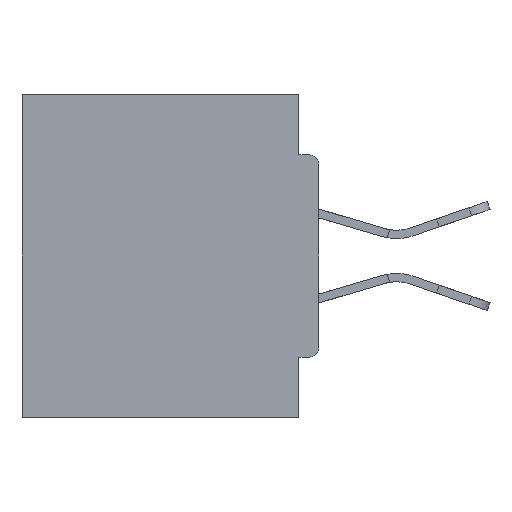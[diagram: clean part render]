
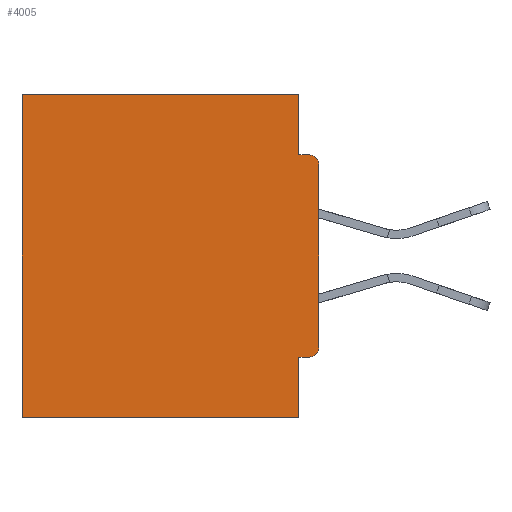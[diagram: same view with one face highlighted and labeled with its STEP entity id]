
A CAD part, left-side view. The second image highlights one B-rep face of the part: STEP entity #4005.
In plain terms, the highlighted planar face has unit normal (-1, 0, 0).
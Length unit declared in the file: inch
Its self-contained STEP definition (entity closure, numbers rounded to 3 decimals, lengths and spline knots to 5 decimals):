
#16 = DIRECTION ( 'NONE',  ( 1., 0., 0. ) ) ;
#240 = CIRCLE ( 'NONE', #25625, 0.015 ) ;
#1523 = LINE ( 'NONE', #36596, #21234 ) ;
#1583 = LINE ( 'NONE', #11855, #23850 ) ;
#2149 = LINE ( 'NONE', #12853, #18045 ) ;
#2560 = DIRECTION ( 'NONE',  ( -1., 0., 0. ) ) ;
#2942 = VERTEX_POINT ( 'NONE', #20227 ) ;
#3557 = CARTESIAN_POINT ( 'NONE',  ( 0.298, 0., 0. ) ) ;
#3755 = VERTEX_POINT ( 'NONE', #22875 ) ;
#3985 = CARTESIAN_POINT ( 'NONE',  ( 0.298, 0.031, -0.4065 ) ) ;
#4005 = ADVANCED_FACE ( 'NONE', ( #28245 ), #24340, .F. ) ;
#4211 = VECTOR ( 'NONE', #34764, 39.37008 ) ;
#5169 = VECTOR ( 'NONE', #29639, 39.37008 ) ;
#5307 = EDGE_CURVE ( 'NONE', #35157, #2942, #1583, .T. ) ;
#5792 = DIRECTION ( 'NONE',  ( 0., 0., -1. ) ) ;
#5953 = EDGE_CURVE ( 'NONE', #29725, #3755, #21306, .T. ) ;
#7488 = ORIENTED_EDGE ( 'NONE', *, *, #39979, .F. ) ;
#9000 = DIRECTION ( 'NONE',  ( 0., 1., 0. ) ) ;
#9446 = ORIENTED_EDGE ( 'NONE', *, *, #5953, .F. ) ;
#9539 = CARTESIAN_POINT ( 'NONE',  ( 0.298, 0.031, -0.5 ) ) ;
#11099 = CARTESIAN_POINT ( 'NONE',  ( 0.298, 0.031, -0.5 ) ) ;
#11128 = EDGE_CURVE ( 'NONE', #38319, #28306, #37104, .T. ) ;
#11855 = CARTESIAN_POINT ( 'NONE',  ( 0.298, 0., -0.5 ) ) ;
#12075 = DIRECTION ( 'NONE',  ( 0., 1., 0. ) ) ;
#12853 = CARTESIAN_POINT ( 'NONE',  ( 0.298, 0.46, 0. ) ) ;
#14094 = VECTOR ( 'NONE', #23771, 39.37008 ) ;
#14181 = VERTEX_POINT ( 'NONE', #31989 ) ;
#14245 = DIRECTION ( 'NONE',  ( -1., 0., 0. ) ) ;
#14380 = ORIENTED_EDGE ( 'NONE', *, *, #28101, .F. ) ;
#14704 = DIRECTION ( 'NONE',  ( 0., 0., -1. ) ) ;
#15812 = ORIENTED_EDGE ( 'NONE', *, *, #5307, .F. ) ;
#16065 = EDGE_CURVE ( 'NONE', #21220, #27363, #38179, .T. ) ;
#16906 = AXIS2_PLACEMENT_3D ( 'NONE', #31310, #2560, #34440 ) ;
#17268 = ORIENTED_EDGE ( 'NONE', *, *, #20866, .F. ) ;
#17435 = ORIENTED_EDGE ( 'NONE', *, *, #24050, .T. ) ;
#18045 = VECTOR ( 'NONE', #28828, 39.37008 ) ;
#18077 = LINE ( 'NONE', #20907, #26802 ) ;
#18659 = LINE ( 'NONE', #11099, #5169 ) ;
#19524 = DIRECTION ( 'NONE',  ( 0., 0., -1. ) ) ;
#19555 = CARTESIAN_POINT ( 'NONE',  ( 0.298, 0., -0.0935 ) ) ;
#20227 = CARTESIAN_POINT ( 'NONE',  ( 0.298, 0.46, -0.5 ) ) ;
#20441 = CARTESIAN_POINT ( 'NONE',  ( 0.298, 0.015, -0.1085 ) ) ;
#20866 = EDGE_CURVE ( 'NONE', #21220, #21267, #1523, .T. ) ;
#20907 = CARTESIAN_POINT ( 'NONE',  ( 0.298, 0.031, -0.5 ) ) ;
#21220 = VERTEX_POINT ( 'NONE', #22187 ) ;
#21234 = VECTOR ( 'NONE', #12075, 39.37008 ) ;
#21267 = VERTEX_POINT ( 'NONE', #3985 ) ;
#21306 = LINE ( 'NONE', #19555, #14094 ) ;
#22187 = CARTESIAN_POINT ( 'NONE',  ( 0.298, 0.015, -0.4065 ) ) ;
#22548 = CARTESIAN_POINT ( 'NONE',  ( 0.298, 0.46, 0. ) ) ;
#22875 = CARTESIAN_POINT ( 'NONE',  ( 0.298, 0.015, -0.0935 ) ) ;
#23253 = ORIENTED_EDGE ( 'NONE', *, *, #16065, .T. ) ;
#23771 = DIRECTION ( 'NONE',  ( 0., -1., 0. ) ) ;
#23850 = VECTOR ( 'NONE', #9000, 39.37008 ) ;
#24050 = EDGE_CURVE ( 'NONE', #14181, #3755, #240, .T. ) ;
#24250 = EDGE_CURVE ( 'NONE', #28306, #2942, #2149, .T. ) ;
#24340 = PLANE ( 'NONE',  #34929 ) ;
#24589 = CARTESIAN_POINT ( 'NONE',  ( 0.298, 0., 0. ) ) ;
#25625 = AXIS2_PLACEMENT_3D ( 'NONE', #20441, #14245, #32651 ) ;
#26802 = VECTOR ( 'NONE', #14704, 39.37008 ) ;
#27363 = VERTEX_POINT ( 'NONE', #29909 ) ;
#27448 = EDGE_LOOP ( 'NONE', ( #17435, #9446, #7488, #31754, #33570, #15812, #14380, #17268, #23253, #27791 ) ) ;
#27791 = ORIENTED_EDGE ( 'NONE', *, *, #33381, .F. ) ;
#28101 = EDGE_CURVE ( 'NONE', #21267, #35157, #18077, .T. ) ;
#28245 = FACE_OUTER_BOUND ( 'NONE', #27448, .T. ) ;
#28306 = VERTEX_POINT ( 'NONE', #22548 ) ;
#28828 = DIRECTION ( 'NONE',  ( 0., 0., -1. ) ) ;
#29639 = DIRECTION ( 'NONE',  ( 0., 0., -1. ) ) ;
#29725 = VERTEX_POINT ( 'NONE', #37715 ) ;
#29909 = CARTESIAN_POINT ( 'NONE',  ( 0.298, 0., -0.3915 ) ) ;
#30298 = VECTOR ( 'NONE', #19524, 39.37008 ) ;
#31310 = CARTESIAN_POINT ( 'NONE',  ( 0.298, 0.015, -0.3915 ) ) ;
#31754 = ORIENTED_EDGE ( 'NONE', *, *, #11128, .T. ) ;
#31989 = CARTESIAN_POINT ( 'NONE',  ( 0.298, 0., -0.1085 ) ) ;
#32079 = CARTESIAN_POINT ( 'NONE',  ( 0.298, 0.031, 0. ) ) ;
#32651 = DIRECTION ( 'NONE',  ( 0., 0., -1. ) ) ;
#32747 = LINE ( 'NONE', #38136, #30298 ) ;
#33381 = EDGE_CURVE ( 'NONE', #14181, #27363, #32747, .T. ) ;
#33570 = ORIENTED_EDGE ( 'NONE', *, *, #24250, .T. ) ;
#34440 = DIRECTION ( 'NONE',  ( 0., 0., -1. ) ) ;
#34764 = DIRECTION ( 'NONE',  ( 0., 1., 0. ) ) ;
#34929 = AXIS2_PLACEMENT_3D ( 'NONE', #24589, #16, #5792 ) ;
#35157 = VERTEX_POINT ( 'NONE', #9539 ) ;
#36596 = CARTESIAN_POINT ( 'NONE',  ( 0.298, 0., -0.4065 ) ) ;
#37104 = LINE ( 'NONE', #3557, #4211 ) ;
#37715 = CARTESIAN_POINT ( 'NONE',  ( 0.298, 0.031, -0.0935 ) ) ;
#38136 = CARTESIAN_POINT ( 'NONE',  ( 0.298, 0., 0. ) ) ;
#38179 = CIRCLE ( 'NONE', #16906, 0.015 ) ;
#38319 = VERTEX_POINT ( 'NONE', #32079 ) ;
#39979 = EDGE_CURVE ( 'NONE', #38319, #29725, #18659, .T. ) ;
